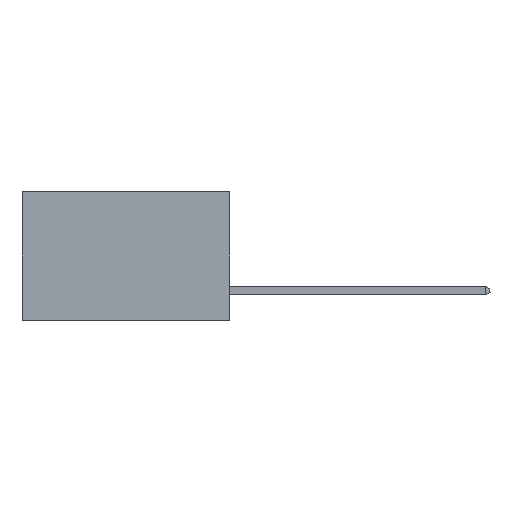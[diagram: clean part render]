
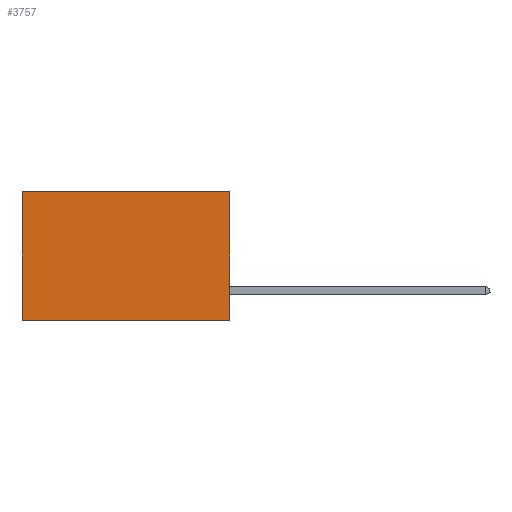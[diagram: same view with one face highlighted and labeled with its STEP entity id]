
A CAD part, left-side view. The second image highlights one B-rep face of the part: STEP entity #3757.
In plain terms, the highlighted planar face has unit normal (-1, 0, 0).
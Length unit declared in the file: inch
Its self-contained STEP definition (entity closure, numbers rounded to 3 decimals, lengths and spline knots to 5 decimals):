
#35 = VERTEX_POINT ( 'NONE', #8280 ) ;
#702 = VERTEX_POINT ( 'NONE', #10543 ) ;
#1143 = DIRECTION ( 'NONE',  ( 0., 0., -1. ) ) ;
#1414 = CARTESIAN_POINT ( 'NONE',  ( 0.298, 0., 0. ) ) ;
#2150 = LINE ( 'NONE', #8204, #11019 ) ;
#2259 = PLANE ( 'NONE',  #6500 ) ;
#2267 = LINE ( 'NONE', #6482, #5550 ) ;
#2453 = EDGE_CURVE ( 'NONE', #702, #35, #2267, .T. ) ;
#2927 = CARTESIAN_POINT ( 'NONE',  ( 0.298, 0., 0. ) ) ;
#3447 = DIRECTION ( 'NONE',  ( 0., 0., -1. ) ) ;
#3557 = DIRECTION ( 'NONE',  ( 1., 0., 0. ) ) ;
#3629 = DIRECTION ( 'NONE',  ( 0., 1., 0. ) ) ;
#3704 = ORIENTED_EDGE ( 'NONE', *, *, #13958, .F. ) ;
#3757 = ADVANCED_FACE ( 'NONE', ( #10931 ), #2259, .F. ) ;
#5550 = VECTOR ( 'NONE', #13160, 39.37008 ) ;
#5743 = CARTESIAN_POINT ( 'NONE',  ( 0.298, 0., 0. ) ) ;
#6482 = CARTESIAN_POINT ( 'NONE',  ( 0.298, 0., -0.37 ) ) ;
#6500 = AXIS2_PLACEMENT_3D ( 'NONE', #5743, #3557, #3447 ) ;
#7806 = VECTOR ( 'NONE', #10420, 39.37008 ) ;
#8005 = ORIENTED_EDGE ( 'NONE', *, *, #2453, .F. ) ;
#8204 = CARTESIAN_POINT ( 'NONE',  ( 0.298, 0.6, 0. ) ) ;
#8241 = EDGE_LOOP ( 'NONE', ( #9041, #8005, #3704, #13430 ) ) ;
#8280 = CARTESIAN_POINT ( 'NONE',  ( 0.298, 0.6, -0.37 ) ) ;
#8385 = LINE ( 'NONE', #1414, #10902 ) ;
#9041 = ORIENTED_EDGE ( 'NONE', *, *, #10792, .T. ) ;
#9265 = CARTESIAN_POINT ( 'NONE',  ( 0.298, 0., 0. ) ) ;
#9627 = VERTEX_POINT ( 'NONE', #12130 ) ;
#10420 = DIRECTION ( 'NONE',  ( 0., 0., -1. ) ) ;
#10543 = CARTESIAN_POINT ( 'NONE',  ( 0.298, 0., -0.37 ) ) ;
#10792 = EDGE_CURVE ( 'NONE', #9627, #35, #2150, .T. ) ;
#10902 = VECTOR ( 'NONE', #3629, 39.37008 ) ;
#10931 = FACE_OUTER_BOUND ( 'NONE', #8241, .T. ) ;
#11019 = VECTOR ( 'NONE', #1143, 39.37008 ) ;
#12130 = CARTESIAN_POINT ( 'NONE',  ( 0.298, 0.6, 0. ) ) ;
#12717 = EDGE_CURVE ( 'NONE', #14808, #9627, #8385, .T. ) ;
#13160 = DIRECTION ( 'NONE',  ( 0., 1., 0. ) ) ;
#13430 = ORIENTED_EDGE ( 'NONE', *, *, #12717, .T. ) ;
#13958 = EDGE_CURVE ( 'NONE', #14808, #702, #14998, .T. ) ;
#14808 = VERTEX_POINT ( 'NONE', #2927 ) ;
#14998 = LINE ( 'NONE', #9265, #7806 ) ;
